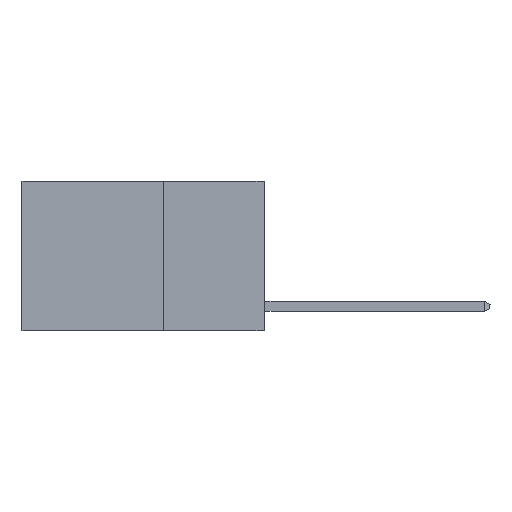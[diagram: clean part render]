
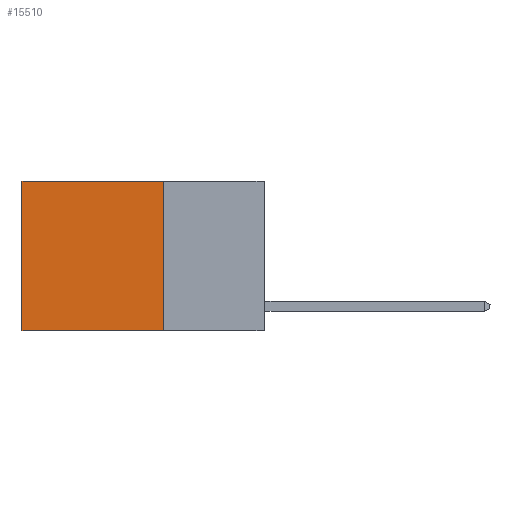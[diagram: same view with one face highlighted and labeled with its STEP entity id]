
A CAD part, left-side view. The second image highlights one B-rep face of the part: STEP entity #15510.
In plain terms, the highlighted planar face has unit normal (-1, 0, 0).
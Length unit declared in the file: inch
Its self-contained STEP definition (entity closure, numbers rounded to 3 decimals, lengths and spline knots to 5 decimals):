
#63 = VERTEX_POINT ( 'NONE', #1547 ) ;
#1547 = CARTESIAN_POINT ( 'NONE',  ( 0.2625, 0.6, -0.37 ) ) ;
#3643 = LINE ( 'NONE', #6712, #5399 ) ;
#5399 = VECTOR ( 'NONE', #13613, 39.37008 ) ;
#5801 = PLANE ( 'NONE',  #26007 ) ;
#5894 = CARTESIAN_POINT ( 'NONE',  ( 0.2625, 0.25, 0. ) ) ;
#6712 = CARTESIAN_POINT ( 'NONE',  ( 0.2625, 0.25, 0. ) ) ;
#7527 = ORIENTED_EDGE ( 'NONE', *, *, #26644, .T. ) ;
#10340 = ORIENTED_EDGE ( 'NONE', *, *, #13256, .F. ) ;
#10488 = DIRECTION ( 'NONE',  ( 0., 0., -1. ) ) ;
#12782 = VERTEX_POINT ( 'NONE', #27921 ) ;
#12869 = EDGE_CURVE ( 'NONE', #27059, #63, #28405, .T. ) ;
#13256 = EDGE_CURVE ( 'NONE', #12782, #27059, #3643, .T. ) ;
#13613 = DIRECTION ( 'NONE',  ( 0., 0., -1. ) ) ;
#13838 = CARTESIAN_POINT ( 'NONE',  ( 0.2625, 0.25, 0. ) ) ;
#14546 = DIRECTION ( 'NONE',  ( 0., 1., 0. ) ) ;
#15457 = VECTOR ( 'NONE', #19832, 39.37008 ) ;
#15510 = ADVANCED_FACE ( 'NONE', ( #29446 ), #5801, .F. ) ;
#16236 = DIRECTION ( 'NONE',  ( 0., 1., 0. ) ) ;
#17745 = CARTESIAN_POINT ( 'NONE',  ( 0.2625, 0.25, -0.37 ) ) ;
#19832 = DIRECTION ( 'NONE',  ( 0., 0., -1. ) ) ;
#20878 = VECTOR ( 'NONE', #14546, 39.37008 ) ;
#21194 = VERTEX_POINT ( 'NONE', #25902 ) ;
#21452 = VECTOR ( 'NONE', #16236, 39.37008 ) ;
#22858 = ORIENTED_EDGE ( 'NONE', *, *, #12869, .F. ) ;
#23715 = CARTESIAN_POINT ( 'NONE',  ( 0.2625, 0.25, -0.37 ) ) ;
#24085 = EDGE_CURVE ( 'NONE', #21194, #63, #26293, .T. ) ;
#24255 = DIRECTION ( 'NONE',  ( 1., 0., 0. ) ) ;
#24339 = CARTESIAN_POINT ( 'NONE',  ( 0.2625, 0.6, 0. ) ) ;
#25902 = CARTESIAN_POINT ( 'NONE',  ( 0.2625, 0.6, 0. ) ) ;
#26007 = AXIS2_PLACEMENT_3D ( 'NONE', #5894, #24255, #10488 ) ;
#26293 = LINE ( 'NONE', #24339, #15457 ) ;
#26644 = EDGE_CURVE ( 'NONE', #12782, #21194, #27548, .T. ) ;
#27059 = VERTEX_POINT ( 'NONE', #17745 ) ;
#27548 = LINE ( 'NONE', #13838, #21452 ) ;
#27726 = EDGE_LOOP ( 'NONE', ( #29610, #22858, #10340, #7527 ) ) ;
#27921 = CARTESIAN_POINT ( 'NONE',  ( 0.2625, 0.25, 0. ) ) ;
#28405 = LINE ( 'NONE', #23715, #20878 ) ;
#29446 = FACE_OUTER_BOUND ( 'NONE', #27726, .T. ) ;
#29610 = ORIENTED_EDGE ( 'NONE', *, *, #24085, .T. ) ;
